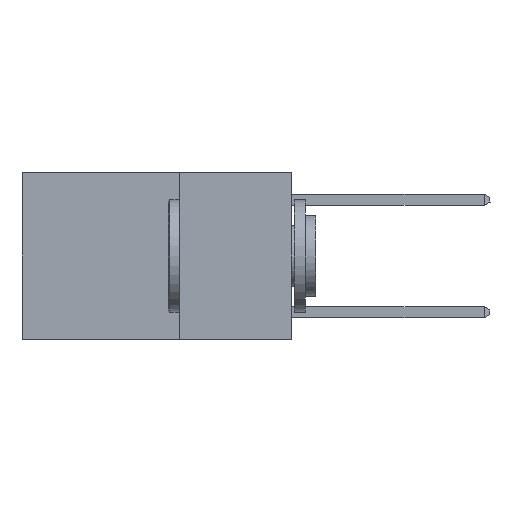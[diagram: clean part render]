
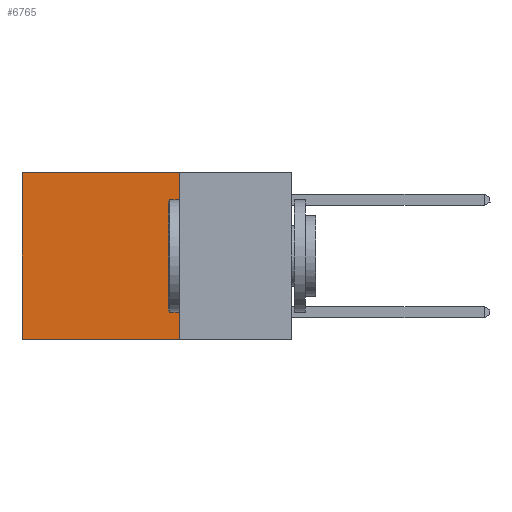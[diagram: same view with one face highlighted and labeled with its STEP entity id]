
A CAD part, left-side view. The second image highlights one B-rep face of the part: STEP entity #6765.
In plain terms, the highlighted planar face has unit normal (-1, 0, 0).
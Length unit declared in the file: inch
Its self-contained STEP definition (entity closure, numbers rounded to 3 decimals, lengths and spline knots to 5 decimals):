
#198 = DIRECTION ( 'NONE',  ( 0., 0., -1. ) ) ;
#1244 = EDGE_CURVE ( 'NONE', #7478, #15494, #11500, .T. ) ;
#2019 = VERTEX_POINT ( 'NONE', #10571 ) ;
#2163 = FACE_OUTER_BOUND ( 'NONE', #2292, .T. ) ;
#2292 = EDGE_LOOP ( 'NONE', ( #2582, #3867, #5515, #13249 ) ) ;
#2582 = ORIENTED_EDGE ( 'NONE', *, *, #13241, .T. ) ;
#2951 = DIRECTION ( 'NONE',  ( 0., 0., -1. ) ) ;
#3703 = VECTOR ( 'NONE', #14404, 39.37008 ) ;
#3867 = ORIENTED_EDGE ( 'NONE', *, *, #9998, .F. ) ;
#4146 = CARTESIAN_POINT ( 'NONE',  ( 0.2625, 0.25, 0. ) ) ;
#5091 = CARTESIAN_POINT ( 'NONE',  ( 0.2625, 0.25, 0. ) ) ;
#5395 = AXIS2_PLACEMENT_3D ( 'NONE', #5091, #7528, #198 ) ;
#5515 = ORIENTED_EDGE ( 'NONE', *, *, #8922, .F. ) ;
#5999 = CARTESIAN_POINT ( 'NONE',  ( 0.2625, 0.25, -0.37 ) ) ;
#6459 = LINE ( 'NONE', #12537, #9668 ) ;
#6542 = CARTESIAN_POINT ( 'NONE',  ( 0.2625, 0.25, 0. ) ) ;
#6765 = ADVANCED_FACE ( 'NONE', ( #2163 ), #9883, .F. ) ;
#6928 = LINE ( 'NONE', #5999, #3703 ) ;
#7478 = VERTEX_POINT ( 'NONE', #4146 ) ;
#7528 = DIRECTION ( 'NONE',  ( 1., 0., 0. ) ) ;
#8922 = EDGE_CURVE ( 'NONE', #7478, #13903, #6459, .T. ) ;
#9668 = VECTOR ( 'NONE', #14880, 39.37008 ) ;
#9883 = PLANE ( 'NONE',  #5395 ) ;
#9998 = EDGE_CURVE ( 'NONE', #13903, #2019, #6928, .T. ) ;
#10047 = DIRECTION ( 'NONE',  ( 0., 1., 0. ) ) ;
#10571 = CARTESIAN_POINT ( 'NONE',  ( 0.2625, 0.6, -0.37 ) ) ;
#11273 = CARTESIAN_POINT ( 'NONE',  ( 0.2625, 0.25, -0.37 ) ) ;
#11396 = CARTESIAN_POINT ( 'NONE',  ( 0.2625, 0.6, 0. ) ) ;
#11500 = LINE ( 'NONE', #6542, #14309 ) ;
#12089 = VECTOR ( 'NONE', #2951, 39.37008 ) ;
#12537 = CARTESIAN_POINT ( 'NONE',  ( 0.2625, 0.25, 0. ) ) ;
#13241 = EDGE_CURVE ( 'NONE', #15494, #2019, #15241, .T. ) ;
#13249 = ORIENTED_EDGE ( 'NONE', *, *, #1244, .T. ) ;
#13903 = VERTEX_POINT ( 'NONE', #11273 ) ;
#14309 = VECTOR ( 'NONE', #10047, 39.37008 ) ;
#14404 = DIRECTION ( 'NONE',  ( 0., 1., 0. ) ) ;
#14880 = DIRECTION ( 'NONE',  ( 0., 0., -1. ) ) ;
#15147 = CARTESIAN_POINT ( 'NONE',  ( 0.2625, 0.6, 0. ) ) ;
#15241 = LINE ( 'NONE', #11396, #12089 ) ;
#15494 = VERTEX_POINT ( 'NONE', #15147 ) ;
